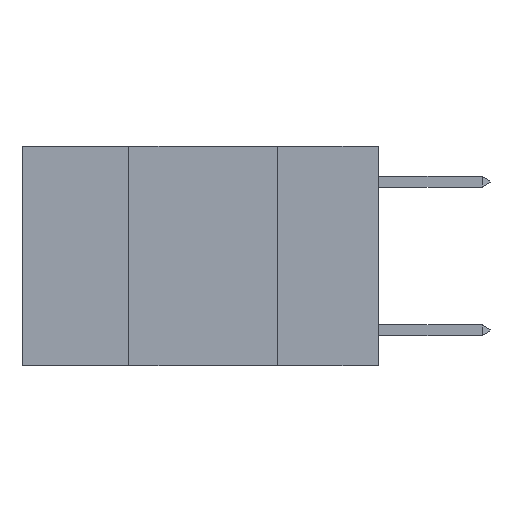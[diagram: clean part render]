
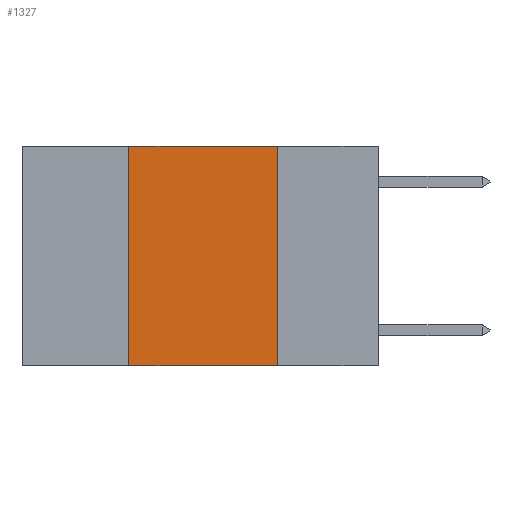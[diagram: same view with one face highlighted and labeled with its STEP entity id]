
A CAD part, left-side view. The second image highlights one B-rep face of the part: STEP entity #1327.
In plain terms, the highlighted planar face has unit normal (-1, 0, 0).
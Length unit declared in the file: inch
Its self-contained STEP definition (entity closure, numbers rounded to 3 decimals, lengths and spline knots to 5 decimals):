
#407 = FACE_OUTER_BOUND ( 'NONE', #12314, .T. ) ;
#591 = DIRECTION ( 'NONE',  ( 0., -1., 0. ) ) ;
#810 = DIRECTION ( 'NONE',  ( 0., 0., 1. ) ) ;
#826 = AXIS2_PLACEMENT_3D ( 'NONE', #11191, #7465, #4822 ) ;
#1176 = ORIENTED_EDGE ( 'NONE', *, *, #13382, .F. ) ;
#1327 = ADVANCED_FACE ( 'NONE', ( #407 ), #10336, .F. ) ;
#1923 = ORIENTED_EDGE ( 'NONE', *, *, #10504, .F. ) ;
#2992 = CARTESIAN_POINT ( 'NONE',  ( 0., 0.17, 0. ) ) ;
#3032 = CARTESIAN_POINT ( 'NONE',  ( 0., 0.6, 0. ) ) ;
#3523 = ORIENTED_EDGE ( 'NONE', *, *, #9731, .T. ) ;
#3710 = VECTOR ( 'NONE', #7355, 39.37008 ) ;
#4362 = LINE ( 'NONE', #13477, #7220 ) ;
#4788 = CARTESIAN_POINT ( 'NONE',  ( 0., 0.6, -0.37 ) ) ;
#4822 = DIRECTION ( 'NONE',  ( 0., 0., -1. ) ) ;
#4914 = VECTOR ( 'NONE', #591, 39.37008 ) ;
#5531 = CARTESIAN_POINT ( 'NONE',  ( 0., 0.17, -0.37 ) ) ;
#5632 = EDGE_CURVE ( 'NONE', #9957, #8048, #9414, .T. ) ;
#7220 = VECTOR ( 'NONE', #810, 39.37008 ) ;
#7355 = DIRECTION ( 'NONE',  ( 0., -1., 0. ) ) ;
#7465 = DIRECTION ( 'NONE',  ( 1., 0., 0. ) ) ;
#8048 = VERTEX_POINT ( 'NONE', #5531 ) ;
#9114 = VERTEX_POINT ( 'NONE', #9200 ) ;
#9200 = CARTESIAN_POINT ( 'NONE',  ( 0., 0.42, 0. ) ) ;
#9414 = LINE ( 'NONE', #12358, #12200 ) ;
#9731 = EDGE_CURVE ( 'NONE', #11417, #8048, #10301, .T. ) ;
#9957 = VERTEX_POINT ( 'NONE', #2992 ) ;
#10301 = LINE ( 'NONE', #4788, #4914 ) ;
#10336 = PLANE ( 'NONE',  #826 ) ;
#10504 = EDGE_CURVE ( 'NONE', #9114, #9957, #12570, .T. ) ;
#10921 = CARTESIAN_POINT ( 'NONE',  ( 0., 0.42, -0.37 ) ) ;
#11191 = CARTESIAN_POINT ( 'NONE',  ( 0., 0.6, 0. ) ) ;
#11417 = VERTEX_POINT ( 'NONE', #10921 ) ;
#11845 = ORIENTED_EDGE ( 'NONE', *, *, #5632, .F. ) ;
#12200 = VECTOR ( 'NONE', #12618, 39.37008 ) ;
#12314 = EDGE_LOOP ( 'NONE', ( #11845, #1923, #1176, #3523 ) ) ;
#12358 = CARTESIAN_POINT ( 'NONE',  ( 0., 0.17, 0. ) ) ;
#12570 = LINE ( 'NONE', #3032, #3710 ) ;
#12618 = DIRECTION ( 'NONE',  ( 0., 0., -1. ) ) ;
#13382 = EDGE_CURVE ( 'NONE', #11417, #9114, #4362, .T. ) ;
#13477 = CARTESIAN_POINT ( 'NONE',  ( 0., 0.42, 0. ) ) ;
